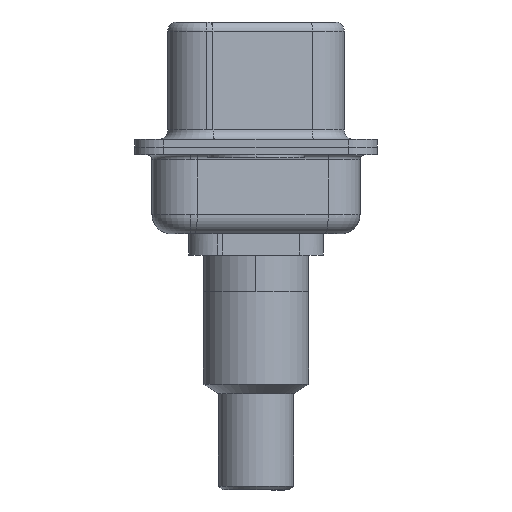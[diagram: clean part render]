
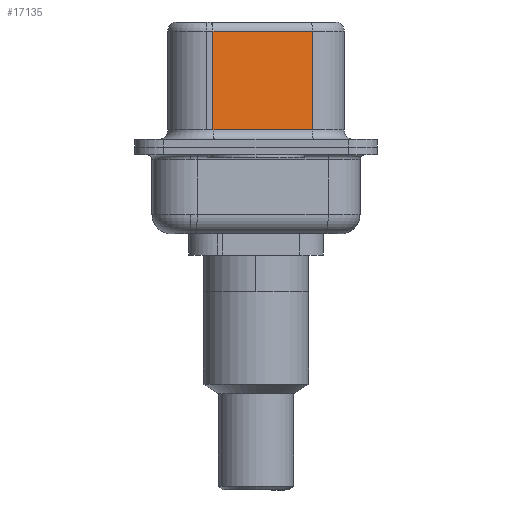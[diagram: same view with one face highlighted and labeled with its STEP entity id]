
A CAD part, left-side view. The second image highlights one B-rep face of the part: STEP entity #17135.
In plain terms, the highlighted planar face has unit normal (-0.985, -0.174, 0).
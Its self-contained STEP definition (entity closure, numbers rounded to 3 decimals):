
#630 = CARTESIAN_POINT ( 'NONE',  ( 3.67, 2.233, 6.02 ) ) ;
#688 = CARTESIAN_POINT ( 'NONE',  ( 4.58, -2.927, 6.52 ) ) ;
#815 = VECTOR ( 'NONE', #3535, 1000. ) ;
#1089 = CARTESIAN_POINT ( 'NONE',  ( 4.58, -2.927, 6.02 ) ) ;
#1604 = EDGE_CURVE ( 'NONE', #13622, #10684, #6146, .T. ) ;
#3216 = DIRECTION ( 'NONE',  ( 0.174, -0.985, 0. ) ) ;
#3318 = EDGE_CURVE ( 'NONE', #12989, #13622, #3742, .T. ) ;
#3535 = DIRECTION ( 'NONE',  ( 0., 0., -1. ) ) ;
#3742 = LINE ( 'NONE', #4788, #815 ) ;
#4272 = LINE ( 'NONE', #688, #15269 ) ;
#4349 = VERTEX_POINT ( 'NONE', #1089 ) ;
#4522 = CARTESIAN_POINT ( 'NONE',  ( 4.58, -2.927, 0.9 ) ) ;
#4598 = AXIS2_PLACEMENT_3D ( 'NONE', #13734, #8253, #5696 ) ;
#4788 = CARTESIAN_POINT ( 'NONE',  ( 3.67, 2.233, 6.52 ) ) ;
#5696 = DIRECTION ( 'NONE',  ( -0.174, 0.985, 0. ) ) ;
#6146 = LINE ( 'NONE', #4522, #8678 ) ;
#6366 = ORIENTED_EDGE ( 'NONE', *, *, #10264, .F. ) ;
#7174 = EDGE_CURVE ( 'NONE', #4349, #12989, #11945, .T. ) ;
#7857 = ORIENTED_EDGE ( 'NONE', *, *, #1604, .T. ) ;
#8253 = DIRECTION ( 'NONE',  ( 0.985, 0.174, 0. ) ) ;
#8678 = VECTOR ( 'NONE', #3216, 1000. ) ;
#9474 = ORIENTED_EDGE ( 'NONE', *, *, #3318, .T. ) ;
#9497 = CARTESIAN_POINT ( 'NONE',  ( 4.58, -2.927, 0.9 ) ) ;
#9953 = FACE_OUTER_BOUND ( 'NONE', #12420, .T. ) ;
#10264 = EDGE_CURVE ( 'NONE', #4349, #10684, #4272, .T. ) ;
#10684 = VERTEX_POINT ( 'NONE', #9497 ) ;
#11945 = LINE ( 'NONE', #13323, #16606 ) ;
#12262 = CARTESIAN_POINT ( 'NONE',  ( 3.67, 2.233, 0.9 ) ) ;
#12420 = EDGE_LOOP ( 'NONE', ( #6366, #16905, #9474, #7857 ) ) ;
#12989 = VERTEX_POINT ( 'NONE', #630 ) ;
#13323 = CARTESIAN_POINT ( 'NONE',  ( 4.58, -2.927, 6.02 ) ) ;
#13622 = VERTEX_POINT ( 'NONE', #12262 ) ;
#13734 = CARTESIAN_POINT ( 'NONE',  ( 4.58, -2.927, 6.52 ) ) ;
#15269 = VECTOR ( 'NONE', #15362, 1000. ) ;
#15362 = DIRECTION ( 'NONE',  ( 0., 0., -1. ) ) ;
#16606 = VECTOR ( 'NONE', #17410, 1000. ) ;
#16905 = ORIENTED_EDGE ( 'NONE', *, *, #7174, .T. ) ;
#17135 = ADVANCED_FACE ( 'NONE', ( #9953 ), #17408, .F. ) ;
#17408 = PLANE ( 'NONE',  #4598 ) ;
#17410 = DIRECTION ( 'NONE',  ( -0.174, 0.985, 0. ) ) ;
